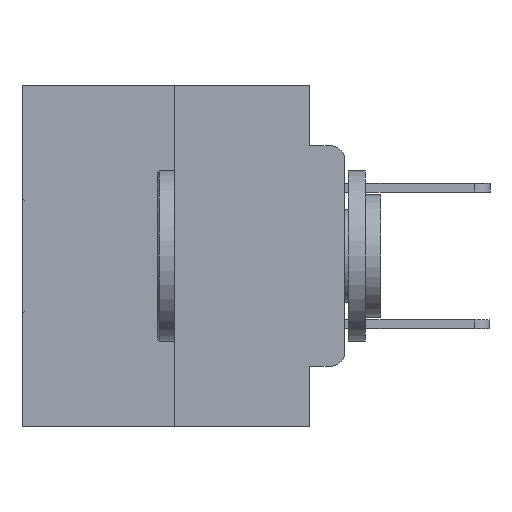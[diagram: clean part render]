
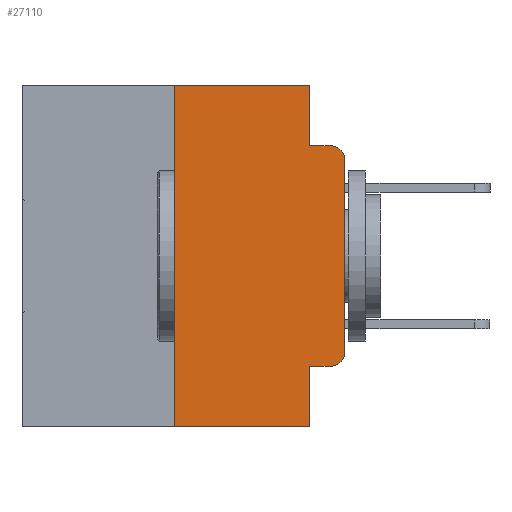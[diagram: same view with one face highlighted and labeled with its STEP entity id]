
A CAD part, left-side view. The second image highlights one B-rep face of the part: STEP entity #27110.
In plain terms, the highlighted planar face has unit normal (-1, 0, 0).
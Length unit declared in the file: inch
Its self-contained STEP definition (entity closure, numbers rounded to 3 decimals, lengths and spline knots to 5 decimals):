
#82 = EDGE_CURVE ( 'NONE', #24517, #21782, #24417, .T. ) ;
#1091 = CARTESIAN_POINT ( 'NONE',  ( 0., 0.473, 0. ) ) ;
#1716 = EDGE_CURVE ( 'NONE', #12850, #14070, #22609, .T. ) ;
#2310 = VECTOR ( 'NONE', #3529, 39.37008 ) ;
#2680 = CIRCLE ( 'NONE', #21454, 0.02 ) ;
#3146 = LINE ( 'NONE', #13658, #15973 ) ;
#3529 = DIRECTION ( 'NONE',  ( 0., -1., 0. ) ) ;
#3589 = ORIENTED_EDGE ( 'NONE', *, *, #29652, .T. ) ;
#3959 = VECTOR ( 'NONE', #24463, 39.37008 ) ;
#4406 = DIRECTION ( 'NONE',  ( -1., 0., 0. ) ) ;
#4467 = DIRECTION ( 'NONE',  ( 0., 0., -1. ) ) ;
#4950 = EDGE_CURVE ( 'NONE', #26862, #14165, #11105, .T. ) ;
#5216 = VECTOR ( 'NONE', #15767, 39.37008 ) ;
#5240 = CARTESIAN_POINT ( 'NONE',  ( 0., 0., -0.1085 ) ) ;
#5283 = CARTESIAN_POINT ( 'NONE',  ( 0., 0.25, 0. ) ) ;
#5349 = EDGE_CURVE ( 'NONE', #12850, #21782, #30578, .T. ) ;
#6034 = CARTESIAN_POINT ( 'NONE',  ( 0., 0.02, -0.0885 ) ) ;
#6202 = ORIENTED_EDGE ( 'NONE', *, *, #6549, .F. ) ;
#6549 = EDGE_CURVE ( 'NONE', #14165, #16510, #3146, .T. ) ;
#6770 = EDGE_CURVE ( 'NONE', #14070, #26862, #15149, .T. ) ;
#6852 = DIRECTION ( 'NONE',  ( 0., -1., 0. ) ) ;
#7003 = CARTESIAN_POINT ( 'NONE',  ( 0., 0., 0. ) ) ;
#7320 = LINE ( 'NONE', #7003, #12999 ) ;
#8153 = EDGE_CURVE ( 'NONE', #21752, #16510, #27785, .T. ) ;
#8603 = CARTESIAN_POINT ( 'NONE',  ( 0., 0.25, 0. ) ) ;
#8913 = DIRECTION ( 'NONE',  ( 0., 0., 1. ) ) ;
#9382 = EDGE_LOOP ( 'NONE', ( #11103, #24655, #6202, #13372, #26155, #26897, #21300, #28360, #3589, #29096 ) ) ;
#9427 = DIRECTION ( 'NONE',  ( 0., 0., 1. ) ) ;
#11103 = ORIENTED_EDGE ( 'NONE', *, *, #11404, .T. ) ;
#11105 = LINE ( 'NONE', #29214, #3959 ) ;
#11404 = EDGE_CURVE ( 'NONE', #30258, #21752, #7320, .T. ) ;
#11651 = CARTESIAN_POINT ( 'NONE',  ( 0., 0.051, 0. ) ) ;
#12850 = VERTEX_POINT ( 'NONE', #13054 ) ;
#12999 = VECTOR ( 'NONE', #9427, 39.37008 ) ;
#13037 = CARTESIAN_POINT ( 'NONE',  ( 0., 0.051, 0. ) ) ;
#13054 = CARTESIAN_POINT ( 'NONE',  ( 0., 0.25, -0.5 ) ) ;
#13180 = DIRECTION ( 'NONE',  ( 0., -1., 0. ) ) ;
#13372 = ORIENTED_EDGE ( 'NONE', *, *, #4950, .F. ) ;
#13658 = CARTESIAN_POINT ( 'NONE',  ( 0., 0.051, -0.0885 ) ) ;
#14070 = VERTEX_POINT ( 'NONE', #5283 ) ;
#14130 = CARTESIAN_POINT ( 'NONE',  ( 0., 0.02, -0.3915 ) ) ;
#14165 = VERTEX_POINT ( 'NONE', #25289 ) ;
#14954 = CARTESIAN_POINT ( 'NONE',  ( 0., 0.051, -0.5 ) ) ;
#15149 = LINE ( 'NONE', #1091, #2310 ) ;
#15165 = VERTEX_POINT ( 'NONE', #26482 ) ;
#15204 = AXIS2_PLACEMENT_3D ( 'NONE', #18836, #4406, #21248 ) ;
#15315 = LINE ( 'NONE', #22748, #27298 ) ;
#15767 = DIRECTION ( 'NONE',  ( 0., 0., -1. ) ) ;
#15973 = VECTOR ( 'NONE', #16104, 39.37008 ) ;
#15998 = CARTESIAN_POINT ( 'NONE',  ( 0., 0.051, -0.4115 ) ) ;
#16104 = DIRECTION ( 'NONE',  ( 0., -1., 0. ) ) ;
#16248 = VECTOR ( 'NONE', #8913, 39.37008 ) ;
#16510 = VERTEX_POINT ( 'NONE', #6034 ) ;
#16567 = DIRECTION ( 'NONE',  ( 0., 0., -1. ) ) ;
#17321 = AXIS2_PLACEMENT_3D ( 'NONE', #23616, #18897, #4467 ) ;
#18836 = CARTESIAN_POINT ( 'NONE',  ( 0., 0.02, -0.1085 ) ) ;
#18897 = DIRECTION ( 'NONE',  ( 1., 0., 0. ) ) ;
#21248 = DIRECTION ( 'NONE',  ( 0., 0., -1. ) ) ;
#21300 = ORIENTED_EDGE ( 'NONE', *, *, #5349, .T. ) ;
#21312 = CARTESIAN_POINT ( 'NONE',  ( 0., 0.473, -0.5 ) ) ;
#21454 = AXIS2_PLACEMENT_3D ( 'NONE', #14130, #30824, #16567 ) ;
#21752 = VERTEX_POINT ( 'NONE', #5240 ) ;
#21782 = VERTEX_POINT ( 'NONE', #14954 ) ;
#22609 = LINE ( 'NONE', #8603, #16248 ) ;
#22748 = CARTESIAN_POINT ( 'NONE',  ( 0., 0.051, -0.4115 ) ) ;
#23299 = EDGE_CURVE ( 'NONE', #15165, #30258, #2680, .T. ) ;
#23616 = CARTESIAN_POINT ( 'NONE',  ( 0., 0.473, 0. ) ) ;
#24291 = VECTOR ( 'NONE', #6852, 39.37008 ) ;
#24417 = LINE ( 'NONE', #11651, #5216 ) ;
#24463 = DIRECTION ( 'NONE',  ( 0., 0., -1. ) ) ;
#24517 = VERTEX_POINT ( 'NONE', #15998 ) ;
#24655 = ORIENTED_EDGE ( 'NONE', *, *, #8153, .T. ) ;
#25289 = CARTESIAN_POINT ( 'NONE',  ( 0., 0.051, -0.0885 ) ) ;
#26155 = ORIENTED_EDGE ( 'NONE', *, *, #6770, .F. ) ;
#26482 = CARTESIAN_POINT ( 'NONE',  ( 0., 0.02, -0.4115 ) ) ;
#26862 = VERTEX_POINT ( 'NONE', #13037 ) ;
#26897 = ORIENTED_EDGE ( 'NONE', *, *, #1716, .F. ) ;
#27110 = ADVANCED_FACE ( 'NONE', ( #30768 ), #30743, .F. ) ;
#27298 = VECTOR ( 'NONE', #13180, 39.37008 ) ;
#27785 = CIRCLE ( 'NONE', #15204, 0.02 ) ;
#28360 = ORIENTED_EDGE ( 'NONE', *, *, #82, .F. ) ;
#28986 = CARTESIAN_POINT ( 'NONE',  ( 0., 0., -0.3915 ) ) ;
#29096 = ORIENTED_EDGE ( 'NONE', *, *, #23299, .T. ) ;
#29214 = CARTESIAN_POINT ( 'NONE',  ( 0., 0.051, 0. ) ) ;
#29652 = EDGE_CURVE ( 'NONE', #24517, #15165, #15315, .T. ) ;
#30258 = VERTEX_POINT ( 'NONE', #28986 ) ;
#30578 = LINE ( 'NONE', #21312, #24291 ) ;
#30743 = PLANE ( 'NONE',  #17321 ) ;
#30768 = FACE_OUTER_BOUND ( 'NONE', #9382, .T. ) ;
#30824 = DIRECTION ( 'NONE',  ( -1., 0., 0. ) ) ;
